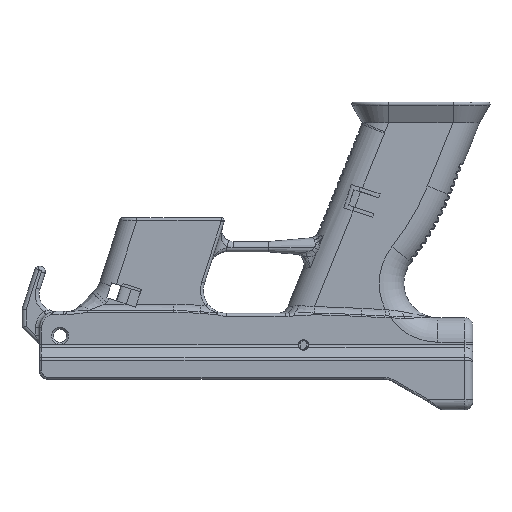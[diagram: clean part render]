
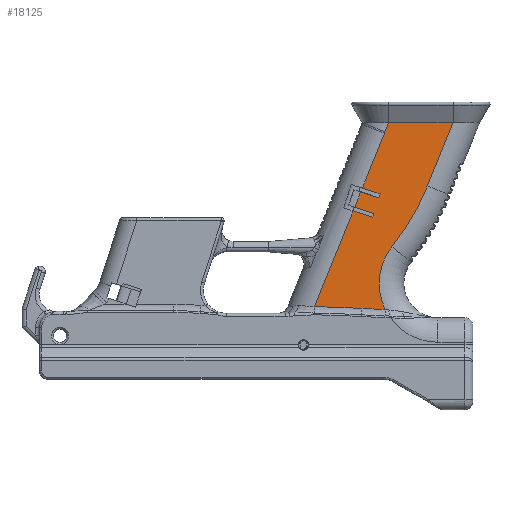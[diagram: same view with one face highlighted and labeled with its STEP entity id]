
A CAD part, front view. The second image highlights one B-rep face of the part: STEP entity #18125.
In plain terms, the highlighted planar face has unit normal (0, -1, 0).
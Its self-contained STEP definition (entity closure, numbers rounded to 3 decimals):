
#2462=FACE_OUTER_BOUND('',#3569,.T.);
#3569=EDGE_LOOP('',(#13965,#13966,#13967,#13968,#13969,#13970,#13971,#13972,
#13973,#13974,#13975,#13976,#13977,#13978,#13979,#13980,#13981));
#4581=CIRCLE('',#19839,696.304);
#4582=CIRCLE('',#19840,689.416);
#4583=CIRCLE('',#19841,28.63);
#4584=CIRCLE('',#19842,118.894);
#4585=CIRCLE('',#19843,17.);
#5493=LINE('',#32775,#6585);
#5508=LINE('',#32915,#6600);
#5509=LINE('',#32923,#6601);
#5551=LINE('',#34583,#6643);
#5552=LINE('',#34585,#6644);
#5553=LINE('',#34586,#6645);
#5554=LINE('',#34595,#6646);
#5555=LINE('',#34597,#6647);
#5556=LINE('',#34600,#6648);
#5557=LINE('',#34602,#6649);
#5558=LINE('',#34604,#6650);
#5559=LINE('',#34605,#6651);
#6585=VECTOR('',#23054,1000.);
#6600=VECTOR('',#23129,1000.);
#6601=VECTOR('',#23136,1000.);
#6643=VECTOR('',#23266,1000.);
#6644=VECTOR('',#23267,1000.);
#6645=VECTOR('',#23268,1000.);
#6646=VECTOR('',#23277,1000.);
#6647=VECTOR('',#23278,1000.);
#6648=VECTOR('',#23281,1000.);
#6649=VECTOR('',#23282,1000.);
#6650=VECTOR('',#23283,1000.);
#6651=VECTOR('',#23284,1000.);
#8251=VERTEX_POINT('',#32740);
#8253=VERTEX_POINT('',#32774);
#8279=VERTEX_POINT('',#32907);
#8280=VERTEX_POINT('',#32914);
#8283=VERTEX_POINT('',#32920);
#8284=VERTEX_POINT('',#32922);
#8366=VERTEX_POINT('',#34581);
#8367=VERTEX_POINT('',#34582);
#8368=VERTEX_POINT('',#34584);
#8369=VERTEX_POINT('',#34587);
#8370=VERTEX_POINT('',#34589);
#8371=VERTEX_POINT('',#34591);
#8372=VERTEX_POINT('',#34594);
#8373=VERTEX_POINT('',#34596);
#8374=VERTEX_POINT('',#34599);
#8375=VERTEX_POINT('',#34601);
#8376=VERTEX_POINT('',#34603);
#10373=EDGE_CURVE('',#8251,#8253,#5493,.T.);
#10415=EDGE_CURVE('',#8279,#8280,#5508,.T.);
#10419=EDGE_CURVE('',#8283,#8284,#5509,.T.);
#10548=EDGE_CURVE('',#8366,#8367,#5551,.T.);
#10549=EDGE_CURVE('',#8366,#8368,#5552,.T.);
#10550=EDGE_CURVE('',#8368,#8280,#5553,.T.);
#10551=EDGE_CURVE('',#8369,#8279,#4581,.T.);
#10552=EDGE_CURVE('',#8370,#8369,#4582,.T.);
#10553=EDGE_CURVE('',#8371,#8370,#4583,.T.);
#10554=EDGE_CURVE('',#8253,#8371,#4584,.T.);
#10555=EDGE_CURVE('',#8372,#8251,#5554,.T.);
#10556=EDGE_CURVE('',#8372,#8373,#5555,.T.);
#10557=EDGE_CURVE('',#8284,#8373,#4585,.T.);
#10558=EDGE_CURVE('',#8283,#8374,#5556,.T.);
#10559=EDGE_CURVE('',#8374,#8375,#5557,.T.);
#10560=EDGE_CURVE('',#8376,#8375,#5558,.T.);
#10561=EDGE_CURVE('',#8367,#8376,#5559,.T.);
#13965=ORIENTED_EDGE('',*,*,#10548,.F.);
#13966=ORIENTED_EDGE('',*,*,#10549,.T.);
#13967=ORIENTED_EDGE('',*,*,#10550,.T.);
#13968=ORIENTED_EDGE('',*,*,#10415,.F.);
#13969=ORIENTED_EDGE('',*,*,#10551,.F.);
#13970=ORIENTED_EDGE('',*,*,#10552,.F.);
#13971=ORIENTED_EDGE('',*,*,#10553,.F.);
#13972=ORIENTED_EDGE('',*,*,#10554,.F.);
#13973=ORIENTED_EDGE('',*,*,#10373,.F.);
#13974=ORIENTED_EDGE('',*,*,#10555,.F.);
#13975=ORIENTED_EDGE('',*,*,#10556,.T.);
#13976=ORIENTED_EDGE('',*,*,#10557,.F.);
#13977=ORIENTED_EDGE('',*,*,#10419,.F.);
#13978=ORIENTED_EDGE('',*,*,#10558,.T.);
#13979=ORIENTED_EDGE('',*,*,#10559,.T.);
#13980=ORIENTED_EDGE('',*,*,#10560,.F.);
#13981=ORIENTED_EDGE('',*,*,#10561,.F.);
#17517=PLANE('',#19838);
#18125=ADVANCED_FACE('',(#2462),#17517,.T.);
#19838=AXIS2_PLACEMENT_3D('',#34580,#23264,#23265);
#19839=AXIS2_PLACEMENT_3D('',#34588,#23269,#23270);
#19840=AXIS2_PLACEMENT_3D('',#34590,#23271,#23272);
#19841=AXIS2_PLACEMENT_3D('',#34592,#23273,#23274);
#19842=AXIS2_PLACEMENT_3D('',#34593,#23275,#23276);
#19843=AXIS2_PLACEMENT_3D('',#34598,#23279,#23280);
#23054=DIRECTION('',(-0.375,0.,-0.927));
#23129=DIRECTION('',(0.375,0.,0.927));
#23136=DIRECTION('',(0.375,0.,0.927));
#23264=DIRECTION('center_axis',(0.,-1.,0.));
#23265=DIRECTION('ref_axis',(0.,0.,-1.));
#23266=DIRECTION('',(-0.952,0.,0.305));
#23267=DIRECTION('',(-0.305,0.,-0.952));
#23268=DIRECTION('',(-0.952,0.,0.305));
#23269=DIRECTION('center_axis',(0.,-1.,0.));
#23270=DIRECTION('ref_axis',(-0.054,0.,-0.999));
#23271=DIRECTION('center_axis',(0.,1.,0.));
#23272=DIRECTION('ref_axis',(0.037,0.,0.999));
#23273=DIRECTION('center_axis',(0.,-1.,0.));
#23274=DIRECTION('ref_axis',(0.782,0.,-0.624));
#23275=DIRECTION('center_axis',(0.,1.,0.));
#23276=DIRECTION('ref_axis',(0.891,0.,-0.454));
#23277=DIRECTION('',(1.,0.,0.));
#23278=DIRECTION('',(-0.375,0.,-0.927));
#23279=DIRECTION('center_axis',(0.,-1.,0.));
#23280=DIRECTION('ref_axis',(0.992,0.,0.126));
#23281=DIRECTION('',(0.952,0.,-0.305));
#23282=DIRECTION('',(-0.305,0.,-0.952));
#23283=DIRECTION('',(0.952,0.,-0.305));
#23284=DIRECTION('',(0.375,0.,0.927));
#32740=CARTESIAN_POINT('',(121.365,-14.625,27.958));
#32774=CARTESIAN_POINT('',(108.893,-14.625,-2.912));
#32775=CARTESIAN_POINT('',(111.761,-14.625,4.188));
#32907=CARTESIAN_POINT('',(53.832,-14.625,-61.703));
#32914=CARTESIAN_POINT('',(72.662,-14.625,-15.097));
#32915=CARTESIAN_POINT('',(70.22,-14.625,-21.141));
#32920=CARTESIAN_POINT('',(77.169,-14.625,-3.94));
#32922=CARTESIAN_POINT('',(87.937,-14.625,22.71));
#32923=CARTESIAN_POINT('',(70.22,-14.625,-21.141));
#34580=CARTESIAN_POINT('Origin',(86.464,-14.625,-15.081));
#34581=CARTESIAN_POINT('',(82.782,-14.625,-16.238));
#34582=CARTESIAN_POINT('',(73.413,-14.625,-13.237));
#34583=CARTESIAN_POINT('',(2.985,-14.625,9.32));
#34584=CARTESIAN_POINT('',(82.172,-14.625,-18.143));
#34585=CARTESIAN_POINT('',(79.797,-14.625,-25.559));
#34586=CARTESIAN_POINT('',(2.375,-14.625,7.416));
#34587=CARTESIAN_POINT('',(76.954,-14.625,-62.561));
#34588=CARTESIAN_POINT('Origin',(39.557,-14.625,-757.86));
#34589=CARTESIAN_POINT('',(88.326,-14.625,-63.079));
#34590=CARTESIAN_POINT('Origin',(113.981,-14.625,625.86));
#34591=CARTESIAN_POINT('',(91.6,-14.625,-32.517));
#34592=CARTESIAN_POINT('Origin',(113.981,-14.625,-50.37));
#34593=CARTESIAN_POINT('Origin',(-1.344,-14.625,41.627));
#34594=CARTESIAN_POINT('',(90.04,-14.625,27.958));
#34595=CARTESIAN_POINT('',(69.665,-14.625,27.958));
#34596=CARTESIAN_POINT('',(88.199,-14.625,23.402));
#34597=CARTESIAN_POINT('',(106.929,-14.625,69.761));
#34598=CARTESIAN_POINT('Origin',(72.175,-14.625,29.078));
#34599=CARTESIAN_POINT('',(85.832,-14.625,-6.715));
#34600=CARTESIAN_POINT('',(88.836,-14.625,-7.677));
#34601=CARTESIAN_POINT('',(85.222,-14.625,-8.619));
#34602=CARTESIAN_POINT('',(79.797,-14.625,-25.559));
#34603=CARTESIAN_POINT('',(76.418,-14.625,-5.799));
#34604=CARTESIAN_POINT('',(88.226,-14.625,-9.581));
#34605=CARTESIAN_POINT('',(70.22,-14.625,-21.141));
